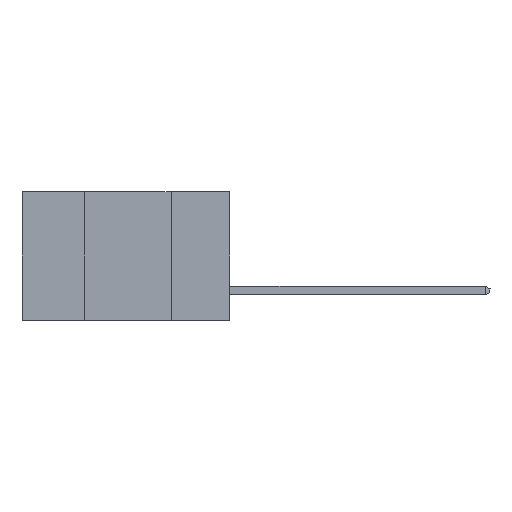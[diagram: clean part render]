
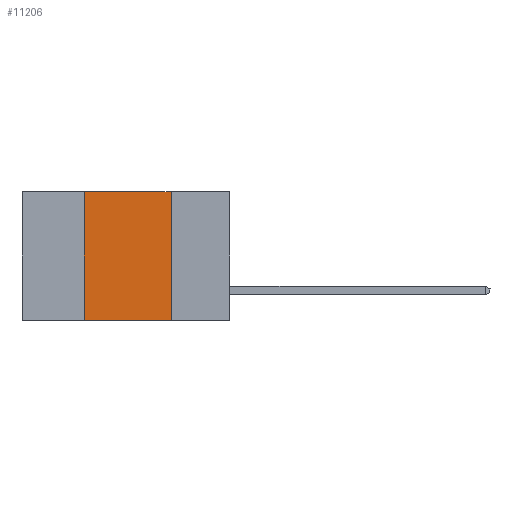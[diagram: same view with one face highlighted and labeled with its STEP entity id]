
A CAD part, left-side view. The second image highlights one B-rep face of the part: STEP entity #11206.
In plain terms, the highlighted planar face has unit normal (-1, 0, 0).
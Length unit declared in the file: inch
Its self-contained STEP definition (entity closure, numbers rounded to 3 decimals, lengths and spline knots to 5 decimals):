
#96 = CARTESIAN_POINT ( 'NONE',  ( 0., 0.42, -0.37 ) ) ;
#190 = PLANE ( 'NONE',  #2161 ) ;
#226 = ORIENTED_EDGE ( 'NONE', *, *, #2406, .T. ) ;
#503 = EDGE_CURVE ( 'NONE', #3265, #9070, #11932, .T. ) ;
#595 = DIRECTION ( 'NONE',  ( 0., -1., 0. ) ) ;
#664 = VERTEX_POINT ( 'NONE', #6469 ) ;
#1126 = EDGE_LOOP ( 'NONE', ( #2858, #1511, #5632, #226 ) ) ;
#1272 = DIRECTION ( 'NONE',  ( 0., 0., -1. ) ) ;
#1371 = VECTOR ( 'NONE', #12259, 39.37008 ) ;
#1511 = ORIENTED_EDGE ( 'NONE', *, *, #11493, .F. ) ;
#1534 = CARTESIAN_POINT ( 'NONE',  ( 0., 0.6, -0.37 ) ) ;
#2161 = AXIS2_PLACEMENT_3D ( 'NONE', #9931, #6076, #1272 ) ;
#2406 = EDGE_CURVE ( 'NONE', #3265, #664, #10077, .T. ) ;
#2858 = ORIENTED_EDGE ( 'NONE', *, *, #8193, .F. ) ;
#3263 = CARTESIAN_POINT ( 'NONE',  ( 0., 0.17, -0.37 ) ) ;
#3265 = VERTEX_POINT ( 'NONE', #96 ) ;
#3307 = CARTESIAN_POINT ( 'NONE',  ( 0., 0.42, -0.37 ) ) ;
#4010 = FACE_OUTER_BOUND ( 'NONE', #1126, .T. ) ;
#4381 = LINE ( 'NONE', #3263, #6278 ) ;
#5314 = DIRECTION ( 'NONE',  ( 0., 0., -1. ) ) ;
#5632 = ORIENTED_EDGE ( 'NONE', *, *, #503, .F. ) ;
#6076 = DIRECTION ( 'NONE',  ( 1., 0., 0. ) ) ;
#6213 = CARTESIAN_POINT ( 'NONE',  ( 0., 0.42, 0. ) ) ;
#6278 = VECTOR ( 'NONE', #5314, 39.37008 ) ;
#6345 = VECTOR ( 'NONE', #595, 39.37008 ) ;
#6469 = CARTESIAN_POINT ( 'NONE',  ( 0., 0.17, -0.37 ) ) ;
#6622 = VECTOR ( 'NONE', #11809, 39.37008 ) ;
#6733 = CARTESIAN_POINT ( 'NONE',  ( 0., 0.17, 0. ) ) ;
#8193 = EDGE_CURVE ( 'NONE', #12220, #664, #4381, .T. ) ;
#9070 = VERTEX_POINT ( 'NONE', #6213 ) ;
#9363 = LINE ( 'NONE', #10376, #1371 ) ;
#9931 = CARTESIAN_POINT ( 'NONE',  ( 0., 0.6, 0. ) ) ;
#10077 = LINE ( 'NONE', #1534, #6345 ) ;
#10376 = CARTESIAN_POINT ( 'NONE',  ( 0., 0.6, 0. ) ) ;
#11206 = ADVANCED_FACE ( 'NONE', ( #4010 ), #190, .F. ) ;
#11493 = EDGE_CURVE ( 'NONE', #9070, #12220, #9363, .T. ) ;
#11809 = DIRECTION ( 'NONE',  ( 0., 0., 1. ) ) ;
#11932 = LINE ( 'NONE', #3307, #6622 ) ;
#12220 = VERTEX_POINT ( 'NONE', #6733 ) ;
#12259 = DIRECTION ( 'NONE',  ( 0., -1., 0. ) ) ;
